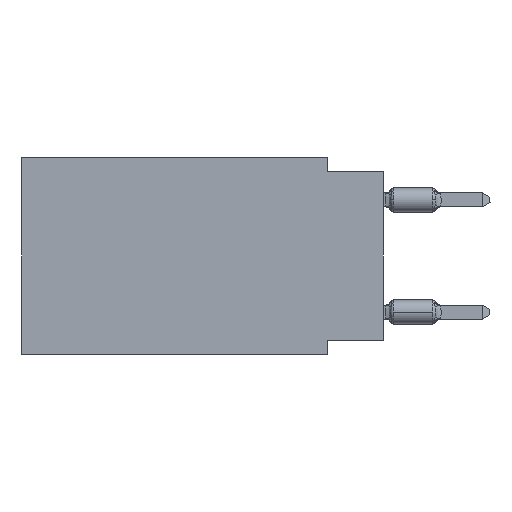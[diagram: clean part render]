
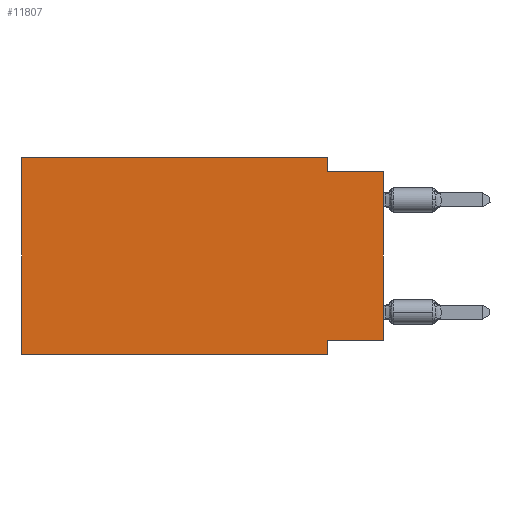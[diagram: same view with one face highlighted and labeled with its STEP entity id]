
A CAD part, left-side view. The second image highlights one B-rep face of the part: STEP entity #11807.
In plain terms, the highlighted planar face has unit normal (-1, 0, 0).
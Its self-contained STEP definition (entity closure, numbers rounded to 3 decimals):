
#339 = EDGE_CURVE ( 'NONE', #15775, #14771, #41894, .T. ) ;
#510 = DIRECTION ( 'NONE',  ( 0., 0., -1. ) ) ;
#1971 = CARTESIAN_POINT ( 'NONE',  ( 0., 16.383, -8.89 ) ) ;
#2015 = CARTESIAN_POINT ( 'NONE',  ( 0., 0., -8.255 ) ) ;
#2179 = CARTESIAN_POINT ( 'NONE',  ( 0., 0., -8.255 ) ) ;
#3085 = EDGE_CURVE ( 'NONE', #5575, #10841, #25856, .T. ) ;
#3282 = CARTESIAN_POINT ( 'NONE',  ( 0., 2.54, 0. ) ) ;
#3284 = VERTEX_POINT ( 'NONE', #31337 ) ;
#4276 = VERTEX_POINT ( 'NONE', #2179 ) ;
#4673 = LINE ( 'NONE', #34222, #34706 ) ;
#5575 = VERTEX_POINT ( 'NONE', #1971 ) ;
#5642 = CARTESIAN_POINT ( 'NONE',  ( 0., 2.54, 0. ) ) ;
#6137 = DIRECTION ( 'NONE',  ( 0., 0., -1. ) ) ;
#6965 = VECTOR ( 'NONE', #510, 1000. ) ;
#7077 = ORIENTED_EDGE ( 'NONE', *, *, #7855, .F. ) ;
#7116 = VECTOR ( 'NONE', #9470, 1000. ) ;
#7342 = DIRECTION ( 'NONE',  ( 0., 0., 1. ) ) ;
#7855 = EDGE_CURVE ( 'NONE', #4276, #31970, #25401, .T. ) ;
#7901 = ORIENTED_EDGE ( 'NONE', *, *, #339, .F. ) ;
#8295 = CARTESIAN_POINT ( 'NONE',  ( 0., 16.383, -8.89 ) ) ;
#8631 = EDGE_CURVE ( 'NONE', #5575, #3284, #37429, .T. ) ;
#8775 = ORIENTED_EDGE ( 'NONE', *, *, #21351, .T. ) ;
#9470 = DIRECTION ( 'NONE',  ( 0., 0., -1. ) ) ;
#10137 = LINE ( 'NONE', #23110, #34187 ) ;
#10841 = VERTEX_POINT ( 'NONE', #15789 ) ;
#11356 = ORIENTED_EDGE ( 'NONE', *, *, #11749, .F. ) ;
#11749 = EDGE_CURVE ( 'NONE', #31970, #3284, #25621, .T. ) ;
#11807 = ADVANCED_FACE ( 'NONE', ( #34856 ), #41248, .F. ) ;
#12358 = VECTOR ( 'NONE', #41047, 1000. ) ;
#12728 = CARTESIAN_POINT ( 'NONE',  ( 0., 2.54, -0.635 ) ) ;
#13740 = EDGE_CURVE ( 'NONE', #10841, #38352, #4673, .T. ) ;
#14111 = VECTOR ( 'NONE', #29046, 1000. ) ;
#14771 = VERTEX_POINT ( 'NONE', #16859 ) ;
#15775 = VERTEX_POINT ( 'NONE', #12728 ) ;
#15789 = CARTESIAN_POINT ( 'NONE',  ( 0., 16.383, 0. ) ) ;
#16859 = CARTESIAN_POINT ( 'NONE',  ( 0., 0., -0.635 ) ) ;
#18188 = DIRECTION ( 'NONE',  ( 0., 1., 0. ) ) ;
#19568 = VECTOR ( 'NONE', #29754, 1000. ) ;
#21063 = DIRECTION ( 'NONE',  ( 0., -1., 0. ) ) ;
#21249 = ORIENTED_EDGE ( 'NONE', *, *, #3085, .F. ) ;
#21351 = EDGE_CURVE ( 'NONE', #4276, #14771, #10137, .T. ) ;
#22417 = CARTESIAN_POINT ( 'NONE',  ( 0., 2.54, -8.255 ) ) ;
#23110 = CARTESIAN_POINT ( 'NONE',  ( 0., 0., 0. ) ) ;
#24653 = ORIENTED_EDGE ( 'NONE', *, *, #13740, .F. ) ;
#25401 = LINE ( 'NONE', #2015, #38806 ) ;
#25621 = LINE ( 'NONE', #38591, #7116 ) ;
#25856 = LINE ( 'NONE', #26461, #14111 ) ;
#26461 = CARTESIAN_POINT ( 'NONE',  ( 0., 16.383, 0. ) ) ;
#26580 = EDGE_LOOP ( 'NONE', ( #8775, #7901, #35679, #24653, #21249, #27626, #11356, #7077 ) ) ;
#27626 = ORIENTED_EDGE ( 'NONE', *, *, #8631, .T. ) ;
#29046 = DIRECTION ( 'NONE',  ( 0., 0., 1. ) ) ;
#29754 = DIRECTION ( 'NONE',  ( 0., -1., 0. ) ) ;
#31337 = CARTESIAN_POINT ( 'NONE',  ( 0., 2.54, -8.89 ) ) ;
#31970 = VERTEX_POINT ( 'NONE', #22417 ) ;
#32431 = LINE ( 'NONE', #3282, #6965 ) ;
#34187 = VECTOR ( 'NONE', #7342, 1000. ) ;
#34222 = CARTESIAN_POINT ( 'NONE',  ( 0., 16.383, 0. ) ) ;
#34650 = CARTESIAN_POINT ( 'NONE',  ( 0., 16.383, 0. ) ) ;
#34706 = VECTOR ( 'NONE', #21063, 1000. ) ;
#34856 = FACE_OUTER_BOUND ( 'NONE', #26580, .T. ) ;
#35679 = ORIENTED_EDGE ( 'NONE', *, *, #36061, .F. ) ;
#36061 = EDGE_CURVE ( 'NONE', #38352, #15775, #32431, .T. ) ;
#37429 = LINE ( 'NONE', #8295, #12358 ) ;
#38352 = VERTEX_POINT ( 'NONE', #5642 ) ;
#38475 = DIRECTION ( 'NONE',  ( 1., 0., 0. ) ) ;
#38591 = CARTESIAN_POINT ( 'NONE',  ( 0., 2.54, -8.89 ) ) ;
#38806 = VECTOR ( 'NONE', #18188, 1000. ) ;
#39312 = CARTESIAN_POINT ( 'NONE',  ( 0., 0., -0.635 ) ) ;
#41047 = DIRECTION ( 'NONE',  ( 0., -1., 0. ) ) ;
#41248 = PLANE ( 'NONE',  #41782 ) ;
#41782 = AXIS2_PLACEMENT_3D ( 'NONE', #34650, #38475, #6137 ) ;
#41894 = LINE ( 'NONE', #39312, #19568 ) ;
